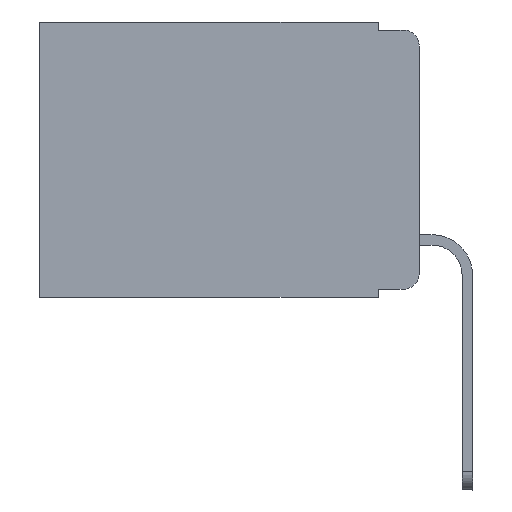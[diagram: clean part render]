
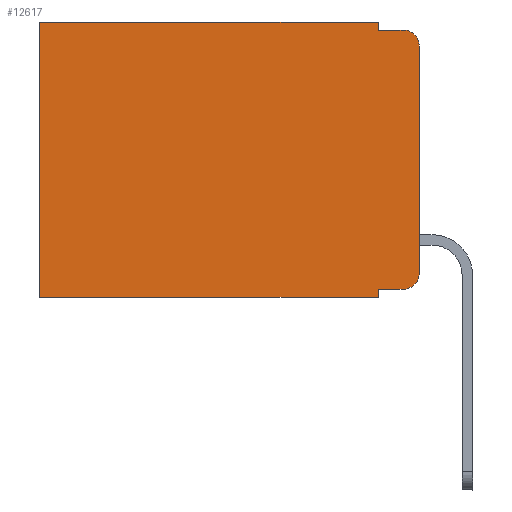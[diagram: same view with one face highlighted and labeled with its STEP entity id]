
A CAD part, left-side view. The second image highlights one B-rep face of the part: STEP entity #12617.
In plain terms, the highlighted planar face has unit normal (-1, 0, 0).
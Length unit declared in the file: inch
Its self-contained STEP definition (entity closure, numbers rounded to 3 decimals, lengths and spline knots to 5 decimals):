
#57 = EDGE_CURVE ( 'NONE', #13437, #4523, #4394, .T. ) ;
#672 = PLANE ( 'NONE',  #10105 ) ;
#745 = CARTESIAN_POINT ( 'NONE',  ( 0.298, 0., 0. ) ) ;
#948 = ORIENTED_EDGE ( 'NONE', *, *, #4544, .F. ) ;
#965 = VERTEX_POINT ( 'NONE', #7991 ) ;
#1176 = EDGE_LOOP ( 'NONE', ( #948, #10665, #4559, #6158, #8977, #13254, #12022, #10094, #5511, #10919 ) ) ;
#1411 = DIRECTION ( 'NONE',  ( 0., 0., -1. ) ) ;
#1842 = CARTESIAN_POINT ( 'NONE',  ( 0.298, 0.051, -0.343 ) ) ;
#1940 = DIRECTION ( 'NONE',  ( 0., 1., 0. ) ) ;
#2096 = EDGE_CURVE ( 'NONE', #4110, #12025, #11291, .T. ) ;
#2185 = DIRECTION ( 'NONE',  ( 0., 0., -1. ) ) ;
#2368 = CARTESIAN_POINT ( 'NONE',  ( 0.298, 0.02, -0.03 ) ) ;
#2737 = DIRECTION ( 'NONE',  ( 0., 0., -1. ) ) ;
#3026 = VECTOR ( 'NONE', #6765, 39.37008 ) ;
#3136 = VECTOR ( 'NONE', #7846, 39.37008 ) ;
#3814 = VECTOR ( 'NONE', #1411, 39.37008 ) ;
#4032 = CARTESIAN_POINT ( 'NONE',  ( 0.298, 0.051, 0. ) ) ;
#4110 = VERTEX_POINT ( 'NONE', #12626 ) ;
#4162 = EDGE_CURVE ( 'NONE', #965, #12575, #13718, .T. ) ;
#4225 = LINE ( 'NONE', #8739, #6532 ) ;
#4394 = LINE ( 'NONE', #12292, #5041 ) ;
#4424 = CARTESIAN_POINT ( 'NONE',  ( 0.298, 0.473, 0. ) ) ;
#4523 = VERTEX_POINT ( 'NONE', #9382 ) ;
#4544 = EDGE_CURVE ( 'NONE', #13936, #5370, #9304, .T. ) ;
#4559 = ORIENTED_EDGE ( 'NONE', *, *, #2096, .F. ) ;
#5041 = VECTOR ( 'NONE', #2185, 39.37008 ) ;
#5241 = DIRECTION ( 'NONE',  ( 0., 0., -1. ) ) ;
#5360 = VERTEX_POINT ( 'NONE', #12649 ) ;
#5370 = VERTEX_POINT ( 'NONE', #7055 ) ;
#5511 = ORIENTED_EDGE ( 'NONE', *, *, #6574, .T. ) ;
#5687 = DIRECTION ( 'NONE',  ( 0., 0., -1. ) ) ;
#6158 = ORIENTED_EDGE ( 'NONE', *, *, #14230, .F. ) ;
#6424 = FACE_OUTER_BOUND ( 'NONE', #1176, .T. ) ;
#6444 = CARTESIAN_POINT ( 'NONE',  ( 0.298, 0., 0. ) ) ;
#6525 = DIRECTION ( 'NONE',  ( 0., 1., 0. ) ) ;
#6532 = VECTOR ( 'NONE', #6525, 39.37008 ) ;
#6574 = EDGE_CURVE ( 'NONE', #965, #5360, #10970, .T. ) ;
#6765 = DIRECTION ( 'NONE',  ( 0., -1., 0. ) ) ;
#6919 = CARTESIAN_POINT ( 'NONE',  ( 0.298, 0., -0.03 ) ) ;
#7055 = CARTESIAN_POINT ( 'NONE',  ( 0.298, 0., -0.313 ) ) ;
#7163 = CARTESIAN_POINT ( 'NONE',  ( 0.298, 0., 0. ) ) ;
#7567 = CARTESIAN_POINT ( 'NONE',  ( 0.298, 0.051, 0. ) ) ;
#7604 = DIRECTION ( 'NONE',  ( 1., 0., 0. ) ) ;
#7846 = DIRECTION ( 'NONE',  ( 0., -1., 0. ) ) ;
#7991 = CARTESIAN_POINT ( 'NONE',  ( 0.298, 0.051, -0.333 ) ) ;
#8509 = DIRECTION ( 'NONE',  ( 0., 0., -1. ) ) ;
#8739 = CARTESIAN_POINT ( 'NONE',  ( 0.298, 0., -0.343 ) ) ;
#8977 = ORIENTED_EDGE ( 'NONE', *, *, #13468, .T. ) ;
#9020 = CARTESIAN_POINT ( 'NONE',  ( 0.298, 0.051, -0.01 ) ) ;
#9079 = DIRECTION ( 'NONE',  ( -1., 0., 0. ) ) ;
#9207 = VECTOR ( 'NONE', #14349, 39.37008 ) ;
#9304 = LINE ( 'NONE', #7163, #3814 ) ;
#9382 = CARTESIAN_POINT ( 'NONE',  ( 0.298, 0.473, -0.343 ) ) ;
#10094 = ORIENTED_EDGE ( 'NONE', *, *, #4162, .F. ) ;
#10105 = AXIS2_PLACEMENT_3D ( 'NONE', #745, #7604, #5241 ) ;
#10665 = ORIENTED_EDGE ( 'NONE', *, *, #12007, .T. ) ;
#10785 = CIRCLE ( 'NONE', #11730, 0.02 ) ;
#10919 = ORIENTED_EDGE ( 'NONE', *, *, #12361, .T. ) ;
#10970 = LINE ( 'NONE', #14424, #3026 ) ;
#10994 = EDGE_CURVE ( 'NONE', #12575, #4523, #4225, .T. ) ;
#11291 = LINE ( 'NONE', #9020, #3136 ) ;
#11372 = DIRECTION ( 'NONE',  ( -1., 0., 0. ) ) ;
#11730 = AXIS2_PLACEMENT_3D ( 'NONE', #2368, #11372, #8509 ) ;
#11852 = LINE ( 'NONE', #4032, #9207 ) ;
#11859 = VERTEX_POINT ( 'NONE', #7567 ) ;
#12007 = EDGE_CURVE ( 'NONE', #13936, #12025, #10785, .T. ) ;
#12022 = ORIENTED_EDGE ( 'NONE', *, *, #10994, .F. ) ;
#12025 = VERTEX_POINT ( 'NONE', #14085 ) ;
#12292 = CARTESIAN_POINT ( 'NONE',  ( 0.298, 0.473, 0. ) ) ;
#12361 = EDGE_CURVE ( 'NONE', #5360, #5370, #13155, .T. ) ;
#12492 = VECTOR ( 'NONE', #2737, 39.37008 ) ;
#12575 = VERTEX_POINT ( 'NONE', #1842 ) ;
#12617 = ADVANCED_FACE ( 'NONE', ( #6424 ), #672, .F. ) ;
#12626 = CARTESIAN_POINT ( 'NONE',  ( 0.298, 0.051, -0.01 ) ) ;
#12649 = CARTESIAN_POINT ( 'NONE',  ( 0.298, 0.02, -0.333 ) ) ;
#12849 = CARTESIAN_POINT ( 'NONE',  ( 0.298, 0.051, 0. ) ) ;
#13145 = AXIS2_PLACEMENT_3D ( 'NONE', #13697, #9079, #5687 ) ;
#13155 = CIRCLE ( 'NONE', #13145, 0.02 ) ;
#13187 = VECTOR ( 'NONE', #1940, 39.37008 ) ;
#13254 = ORIENTED_EDGE ( 'NONE', *, *, #57, .T. ) ;
#13279 = LINE ( 'NONE', #6444, #13187 ) ;
#13437 = VERTEX_POINT ( 'NONE', #4424 ) ;
#13468 = EDGE_CURVE ( 'NONE', #11859, #13437, #13279, .T. ) ;
#13697 = CARTESIAN_POINT ( 'NONE',  ( 0.298, 0.02, -0.313 ) ) ;
#13718 = LINE ( 'NONE', #12849, #12492 ) ;
#13936 = VERTEX_POINT ( 'NONE', #6919 ) ;
#14085 = CARTESIAN_POINT ( 'NONE',  ( 0.298, 0.02, -0.01 ) ) ;
#14230 = EDGE_CURVE ( 'NONE', #11859, #4110, #11852, .T. ) ;
#14349 = DIRECTION ( 'NONE',  ( 0., 0., -1. ) ) ;
#14424 = CARTESIAN_POINT ( 'NONE',  ( 0.298, 0.051, -0.333 ) ) ;
